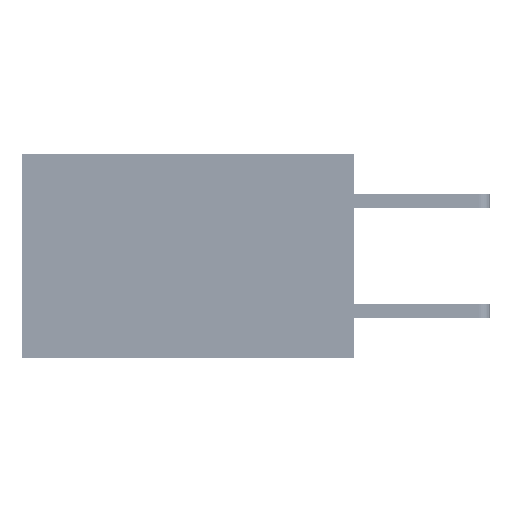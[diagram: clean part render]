
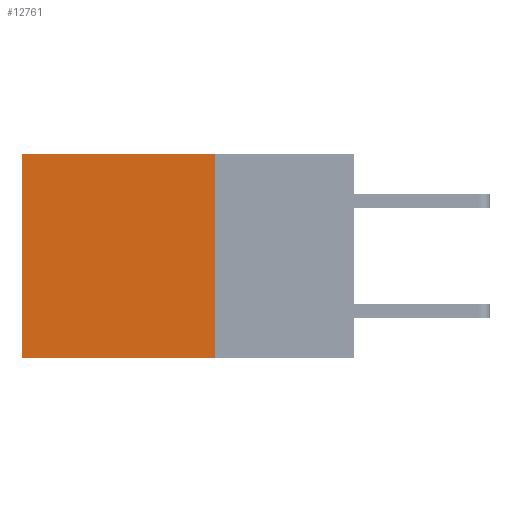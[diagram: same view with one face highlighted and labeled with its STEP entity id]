
A CAD part, left-side view. The second image highlights one B-rep face of the part: STEP entity #12761.
In plain terms, the highlighted planar face has unit normal (-1, 0, 0).
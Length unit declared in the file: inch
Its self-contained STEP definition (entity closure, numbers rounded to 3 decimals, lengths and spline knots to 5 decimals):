
#1325 = DIRECTION ( 'NONE',  ( 0., 0., -1. ) ) ;
#1366 = CARTESIAN_POINT ( 'NONE',  ( 0.2875, 0.6, 0. ) ) ;
#2367 = ORIENTED_EDGE ( 'NONE', *, *, #27090, .F. ) ;
#2371 = LINE ( 'NONE', #39985, #27963 ) ;
#2567 = FACE_OUTER_BOUND ( 'NONE', #35594, .T. ) ;
#2960 = LINE ( 'NONE', #27131, #29988 ) ;
#3733 = VERTEX_POINT ( 'NONE', #24614 ) ;
#4308 = ORIENTED_EDGE ( 'NONE', *, *, #22033, .F. ) ;
#4509 = EDGE_CURVE ( 'NONE', #19484, #3733, #2960, .T. ) ;
#8150 = ORIENTED_EDGE ( 'NONE', *, *, #4509, .T. ) ;
#8315 = DIRECTION ( 'NONE',  ( 0., 1., 0. ) ) ;
#10808 = DIRECTION ( 'NONE',  ( 1., 0., 0. ) ) ;
#12212 = AXIS2_PLACEMENT_3D ( 'NONE', #38708, #10808, #1325 ) ;
#12761 = ADVANCED_FACE ( 'NONE', ( #2567 ), #29452, .F. ) ;
#13906 = EDGE_CURVE ( 'NONE', #3733, #16738, #32574, .T. ) ;
#16738 = VERTEX_POINT ( 'NONE', #26038 ) ;
#18580 = DIRECTION ( 'NONE',  ( 0., 1., 0. ) ) ;
#19484 = VERTEX_POINT ( 'NONE', #24082 ) ;
#22033 = EDGE_CURVE ( 'NONE', #19484, #37883, #2371, .T. ) ;
#24082 = CARTESIAN_POINT ( 'NONE',  ( 0.2875, 0.25, 0. ) ) ;
#24614 = CARTESIAN_POINT ( 'NONE',  ( 0.2875, 0.6, 0. ) ) ;
#26038 = CARTESIAN_POINT ( 'NONE',  ( 0.2875, 0.6, -0.37 ) ) ;
#27090 = EDGE_CURVE ( 'NONE', #37883, #16738, #30151, .T. ) ;
#27131 = CARTESIAN_POINT ( 'NONE',  ( 0.2875, 0.25, 0. ) ) ;
#27492 = DIRECTION ( 'NONE',  ( 0., 0., -1. ) ) ;
#27963 = VECTOR ( 'NONE', #27492, 39.37008 ) ;
#28810 = ORIENTED_EDGE ( 'NONE', *, *, #13906, .T. ) ;
#29452 = PLANE ( 'NONE',  #12212 ) ;
#29988 = VECTOR ( 'NONE', #8315, 39.37008 ) ;
#30151 = LINE ( 'NONE', #37331, #37073 ) ;
#32574 = LINE ( 'NONE', #1366, #37987 ) ;
#35594 = EDGE_LOOP ( 'NONE', ( #28810, #2367, #4308, #8150 ) ) ;
#36696 = DIRECTION ( 'NONE',  ( 0., 0., -1. ) ) ;
#37073 = VECTOR ( 'NONE', #18580, 39.37008 ) ;
#37331 = CARTESIAN_POINT ( 'NONE',  ( 0.2875, 0.25, -0.37 ) ) ;
#37883 = VERTEX_POINT ( 'NONE', #39752 ) ;
#37987 = VECTOR ( 'NONE', #36696, 39.37008 ) ;
#38708 = CARTESIAN_POINT ( 'NONE',  ( 0.2875, 0.25, 0. ) ) ;
#39752 = CARTESIAN_POINT ( 'NONE',  ( 0.2875, 0.25, -0.37 ) ) ;
#39985 = CARTESIAN_POINT ( 'NONE',  ( 0.2875, 0.25, 0. ) ) ;
